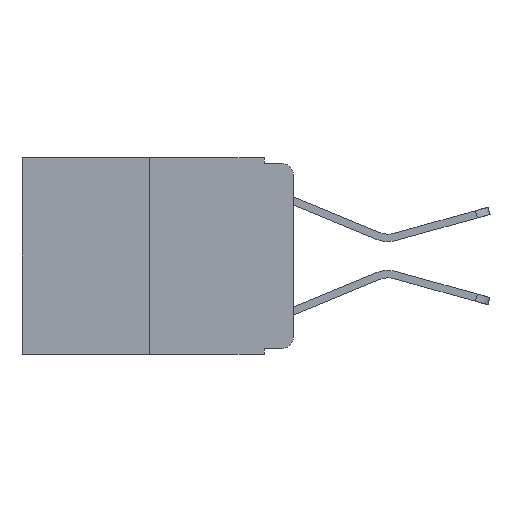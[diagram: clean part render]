
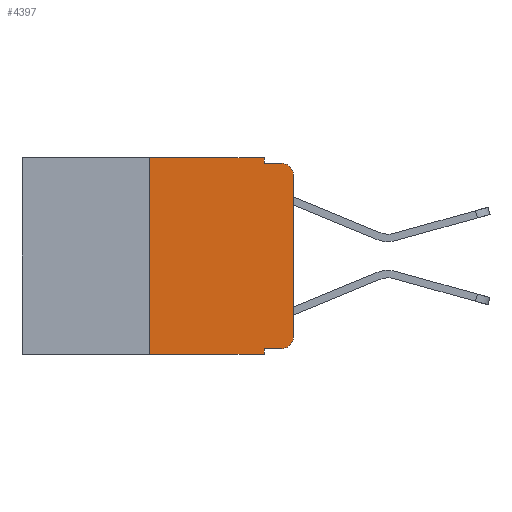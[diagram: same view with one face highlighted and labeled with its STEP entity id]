
A CAD part, left-side view. The second image highlights one B-rep face of the part: STEP entity #4397.
In plain terms, the highlighted planar face has unit normal (-1, 0, 0).
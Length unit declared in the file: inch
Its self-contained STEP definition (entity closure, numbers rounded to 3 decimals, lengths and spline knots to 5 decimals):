
#164 = DIRECTION ( 'NONE',  ( 1., 0., 0. ) ) ;
#178 = AXIS2_PLACEMENT_3D ( 'NONE', #8558, #164, #9941 ) ;
#429 = DIRECTION ( 'NONE',  ( 0., 0., -1. ) ) ;
#861 = VERTEX_POINT ( 'NONE', #16680 ) ;
#1368 = AXIS2_PLACEMENT_3D ( 'NONE', #15488, #7363, #16730 ) ;
#1820 = DIRECTION ( 'NONE',  ( 0., -1., 0. ) ) ;
#2520 = CARTESIAN_POINT ( 'NONE',  ( 0., 0.473, -0.343 ) ) ;
#2560 = VERTEX_POINT ( 'NONE', #10452 ) ;
#3067 = EDGE_LOOP ( 'NONE', ( #9729, #13336, #6566, #13745, #17152, #6979, #10594, #3764, #7378, #14594 ) ) ;
#3227 = CARTESIAN_POINT ( 'NONE',  ( 0., 0.051, -0.01 ) ) ;
#3764 = ORIENTED_EDGE ( 'NONE', *, *, #9696, .F. ) ;
#3870 = CARTESIAN_POINT ( 'NONE',  ( 0., 0.051, -0.01 ) ) ;
#3998 = DIRECTION ( 'NONE',  ( 0., -1., 0. ) ) ;
#4243 = CIRCLE ( 'NONE', #17133, 0.02 ) ;
#4397 = ADVANCED_FACE ( 'NONE', ( #6905 ), #15302, .F. ) ;
#4662 = DIRECTION ( 'NONE',  ( 0., -1., 0. ) ) ;
#4676 = VECTOR ( 'NONE', #7428, 39.37008 ) ;
#4838 = DIRECTION ( 'NONE',  ( -1., 0., 0. ) ) ;
#5320 = CARTESIAN_POINT ( 'NONE',  ( 0., 0.473, 0. ) ) ;
#5507 = LINE ( 'NONE', #6100, #4676 ) ;
#5637 = VERTEX_POINT ( 'NONE', #8635 ) ;
#6029 = DIRECTION ( 'NONE',  ( 0., 0., -1. ) ) ;
#6100 = CARTESIAN_POINT ( 'NONE',  ( 0., 0.25, 0. ) ) ;
#6332 = CARTESIAN_POINT ( 'NONE',  ( 0., 0.02, -0.01 ) ) ;
#6438 = VERTEX_POINT ( 'NONE', #13311 ) ;
#6566 = ORIENTED_EDGE ( 'NONE', *, *, #9665, .F. ) ;
#6905 = FACE_OUTER_BOUND ( 'NONE', #3067, .T. ) ;
#6979 = ORIENTED_EDGE ( 'NONE', *, *, #9693, .F. ) ;
#7363 = DIRECTION ( 'NONE',  ( -1., 0., 0. ) ) ;
#7378 = ORIENTED_EDGE ( 'NONE', *, *, #9719, .T. ) ;
#7428 = DIRECTION ( 'NONE',  ( 0., 0., 1. ) ) ;
#7429 = VECTOR ( 'NONE', #3998, 39.37008 ) ;
#7442 = LINE ( 'NONE', #5320, #11504 ) ;
#7641 = CARTESIAN_POINT ( 'NONE',  ( 0., 0.02, -0.333 ) ) ;
#7840 = VECTOR ( 'NONE', #1820, 39.37008 ) ;
#8262 = LINE ( 'NONE', #8793, #7840 ) ;
#8558 = CARTESIAN_POINT ( 'NONE',  ( 0., 0.473, 0. ) ) ;
#8617 = DIRECTION ( 'NONE',  ( 0., 0., 1. ) ) ;
#8635 = CARTESIAN_POINT ( 'NONE',  ( 0., 0.051, -0.333 ) ) ;
#8697 = VECTOR ( 'NONE', #6029, 39.37008 ) ;
#8793 = CARTESIAN_POINT ( 'NONE',  ( 0., 0.051, -0.333 ) ) ;
#8876 = VERTEX_POINT ( 'NONE', #7641 ) ;
#9009 = EDGE_CURVE ( 'NONE', #16141, #10875, #7442, .T. ) ;
#9117 = VECTOR ( 'NONE', #4662, 39.37008 ) ;
#9417 = EDGE_CURVE ( 'NONE', #11570, #6438, #14634, .T. ) ;
#9634 = EDGE_CURVE ( 'NONE', #2560, #861, #16650, .T. ) ;
#9663 = EDGE_CURVE ( 'NONE', #861, #10782, #12744, .T. ) ;
#9665 = EDGE_CURVE ( 'NONE', #15999, #10782, #15895, .T. ) ;
#9670 = EDGE_CURVE ( 'NONE', #10875, #15999, #12327, .T. ) ;
#9693 = EDGE_CURVE ( 'NONE', #11570, #16141, #5507, .T. ) ;
#9696 = EDGE_CURVE ( 'NONE', #5637, #6438, #15474, .T. ) ;
#9719 = EDGE_CURVE ( 'NONE', #5637, #8876, #8262, .T. ) ;
#9723 = EDGE_CURVE ( 'NONE', #8876, #2560, #4243, .T. ) ;
#9729 = ORIENTED_EDGE ( 'NONE', *, *, #9634, .T. ) ;
#9772 = CARTESIAN_POINT ( 'NONE',  ( 0., 0.25, -0.343 ) ) ;
#9941 = DIRECTION ( 'NONE',  ( 0., 0., -1. ) ) ;
#9985 = VECTOR ( 'NONE', #8617, 39.37008 ) ;
#10452 = CARTESIAN_POINT ( 'NONE',  ( 0., 0., -0.313 ) ) ;
#10594 = ORIENTED_EDGE ( 'NONE', *, *, #9417, .T. ) ;
#10782 = VERTEX_POINT ( 'NONE', #6332 ) ;
#10875 = VERTEX_POINT ( 'NONE', #17121 ) ;
#11138 = CARTESIAN_POINT ( 'NONE',  ( 0., 0.25, 0. ) ) ;
#11368 = CARTESIAN_POINT ( 'NONE',  ( 0., 0., 0. ) ) ;
#11504 = VECTOR ( 'NONE', #14796, 39.37008 ) ;
#11570 = VERTEX_POINT ( 'NONE', #9772 ) ;
#12327 = LINE ( 'NONE', #16683, #8697 ) ;
#12744 = CIRCLE ( 'NONE', #1368, 0.02 ) ;
#12972 = CARTESIAN_POINT ( 'NONE',  ( 0., 0.02, -0.313 ) ) ;
#13311 = CARTESIAN_POINT ( 'NONE',  ( 0., 0.051, -0.343 ) ) ;
#13336 = ORIENTED_EDGE ( 'NONE', *, *, #9663, .T. ) ;
#13745 = ORIENTED_EDGE ( 'NONE', *, *, #9670, .F. ) ;
#14309 = DIRECTION ( 'NONE',  ( 0., 0., -1. ) ) ;
#14594 = ORIENTED_EDGE ( 'NONE', *, *, #9723, .T. ) ;
#14634 = LINE ( 'NONE', #2520, #7429 ) ;
#14796 = DIRECTION ( 'NONE',  ( 0., -1., 0. ) ) ;
#15039 = VECTOR ( 'NONE', #429, 39.37008 ) ;
#15302 = PLANE ( 'NONE',  #178 ) ;
#15474 = LINE ( 'NONE', #15541, #15039 ) ;
#15488 = CARTESIAN_POINT ( 'NONE',  ( 0., 0.02, -0.03 ) ) ;
#15541 = CARTESIAN_POINT ( 'NONE',  ( 0., 0.051, 0. ) ) ;
#15895 = LINE ( 'NONE', #3227, #9117 ) ;
#15999 = VERTEX_POINT ( 'NONE', #3870 ) ;
#16141 = VERTEX_POINT ( 'NONE', #11138 ) ;
#16650 = LINE ( 'NONE', #11368, #9985 ) ;
#16680 = CARTESIAN_POINT ( 'NONE',  ( 0., 0., -0.03 ) ) ;
#16683 = CARTESIAN_POINT ( 'NONE',  ( 0., 0.051, 0. ) ) ;
#16730 = DIRECTION ( 'NONE',  ( 0., 0., -1. ) ) ;
#17121 = CARTESIAN_POINT ( 'NONE',  ( 0., 0.051, 0. ) ) ;
#17133 = AXIS2_PLACEMENT_3D ( 'NONE', #12972, #4838, #14309 ) ;
#17152 = ORIENTED_EDGE ( 'NONE', *, *, #9009, .F. ) ;
